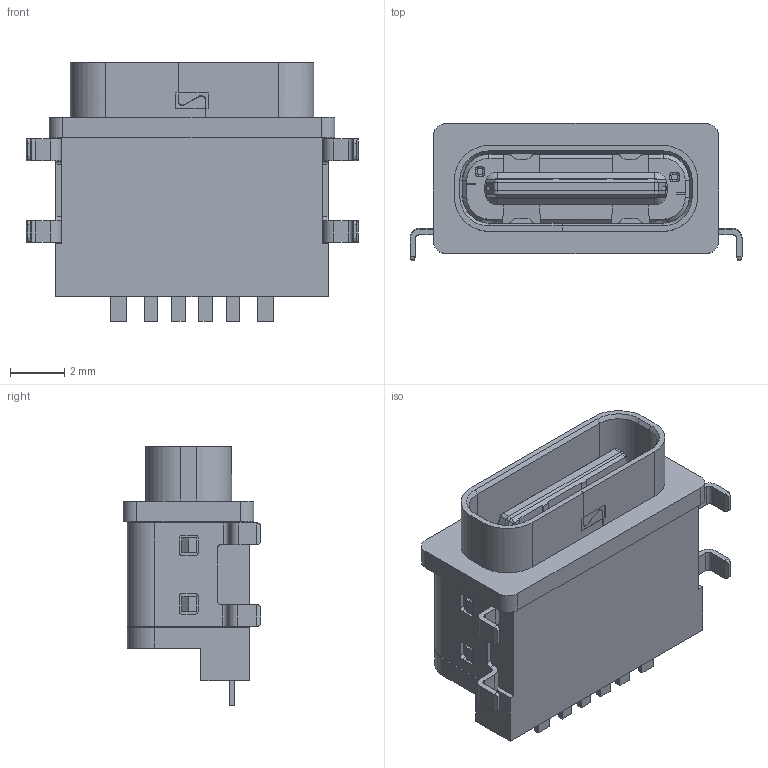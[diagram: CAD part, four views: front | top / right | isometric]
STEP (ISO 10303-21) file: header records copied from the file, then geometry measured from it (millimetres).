
FILE_DESCRIPTION (( 'STEP AP214' ), '1' );
FILE_NAME ('698A106W182-611.STEP', '2021-01-15T12:48:13', ( '' ), ( '' ), 'SwSTEP 2.0', 'SolidWorks 2020', '' );
FILE_SCHEMA (( 'AUTOMOTIVE_DESIGN' ));
Length unit declared in the file: millimetre
Products named in the file (7): Insulator2 698A106WX82-611; 698A106W182-611; Shell1 698A106WX82-611; Housing 698A106WX82-611; Insulator 698A106WX82-611; Shell2 698A106WX82-611; Contacts 698A106WX82-611
Assembly tree (6 placements, depth 2):
  698A106W182-611
    Insulator 698A106WX82-611
    Contacts 698A106WX82-611
    Shell1 698A106WX82-611
    Shell2 698A106WX82-611
    Housing 698A106WX82-611
    Insulator2 698A106WX82-611
Bounding box: 12.2 x 5.05 x 9.5 mm (x, y, z)
Volume: 234.6 mm3; surface area: 1160.6 mm2
Topology: 11 solids, 11 shells, 1276 faces, 3514 edges, 2303 vertices
Faces by surface type: plane 896, cylinder 329, cone 29, bspline 22
Entity records: 41232 total; most frequent: CARTESIAN_POINT 8123, ORIENTED_EDGE 7020, DIRECTION 6585, EDGE_CURVE 3510, LINE 2727, VECTOR 2727, VERTEX_POINT 2303, AXIS2_PLACEMENT_3D 1929
